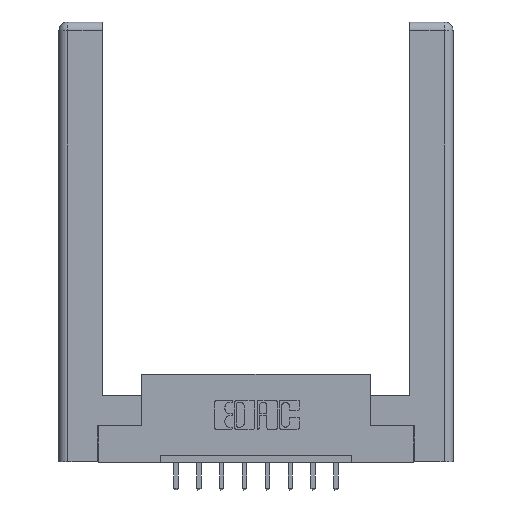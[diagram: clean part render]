
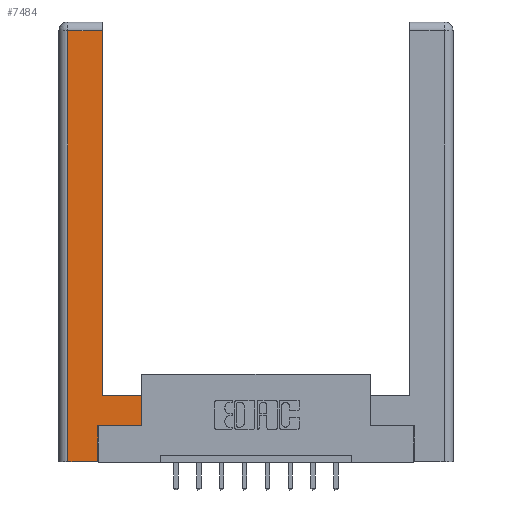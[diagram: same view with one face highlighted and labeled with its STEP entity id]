
A CAD part, top view. The second image highlights one B-rep face of the part: STEP entity #7484.
In plain terms, the highlighted planar face has unit normal (0, 0, 1).
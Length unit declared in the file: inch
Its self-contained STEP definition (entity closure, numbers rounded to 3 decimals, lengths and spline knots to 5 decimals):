
#339 = CARTESIAN_POINT ( 'NONE',  ( 0.295, 3., 0. ) ) ;
#538 = VERTEX_POINT ( 'NONE', #12807 ) ;
#664 = ORIENTED_EDGE ( 'NONE', *, *, #1792, .T. ) ;
#1114 = VERTEX_POINT ( 'NONE', #7267 ) ;
#1497 = EDGE_CURVE ( 'NONE', #6639, #1114, #12967, .T. ) ;
#1628 = EDGE_CURVE ( 'NONE', #7565, #3697, #8568, .T. ) ;
#1708 = VECTOR ( 'NONE', #4663, 39.37008 ) ;
#1780 = CARTESIAN_POINT ( 'NONE',  ( 0.0615, 0., 0. ) ) ;
#1792 = EDGE_CURVE ( 'NONE', #10190, #4879, #8413, .T. ) ;
#1850 = CARTESIAN_POINT ( 'NONE',  ( 0.295, 0.45, 0. ) ) ;
#1873 = VECTOR ( 'NONE', #5642, 39.37008 ) ;
#1914 = DIRECTION ( 'NONE',  ( 0., -1., 0. ) ) ;
#2356 = VECTOR ( 'NONE', #4478, 39.37008 ) ;
#2445 = VECTOR ( 'NONE', #11176, 39.37008 ) ;
#2624 = CARTESIAN_POINT ( 'NONE',  ( 0.565, 0.245, 0. ) ) ;
#2891 = ORIENTED_EDGE ( 'NONE', *, *, #10321, .T. ) ;
#2970 = DIRECTION ( 'NONE',  ( 0., 0., -1. ) ) ;
#3054 = CARTESIAN_POINT ( 'NONE',  ( 0.0615, 2.94, 0. ) ) ;
#3135 = LINE ( 'NONE', #2624, #1708 ) ;
#3470 = CARTESIAN_POINT ( 'NONE',  ( 0.265, 0., 0. ) ) ;
#3697 = VERTEX_POINT ( 'NONE', #6458 ) ;
#3754 = EDGE_CURVE ( 'NONE', #3697, #10190, #5165, .T. ) ;
#3959 = ORIENTED_EDGE ( 'NONE', *, *, #4753, .T. ) ;
#4136 = EDGE_LOOP ( 'NONE', ( #6158, #7349, #664, #9081, #11335, #2891, #3959, #4630 ) ) ;
#4271 = CARTESIAN_POINT ( 'NONE',  ( 0.0615, 2.94, 0. ) ) ;
#4478 = DIRECTION ( 'NONE',  ( -1., 0., 0. ) ) ;
#4630 = ORIENTED_EDGE ( 'NONE', *, *, #10845, .T. ) ;
#4663 = DIRECTION ( 'NONE',  ( 1., 0., 0. ) ) ;
#4753 = EDGE_CURVE ( 'NONE', #538, #11737, #5563, .T. ) ;
#4879 = VERTEX_POINT ( 'NONE', #10035 ) ;
#5082 = VECTOR ( 'NONE', #11844, 39.37008 ) ;
#5165 = LINE ( 'NONE', #3054, #2445 ) ;
#5563 = LINE ( 'NONE', #10769, #1873 ) ;
#5642 = DIRECTION ( 'NONE',  ( 0., 1., 0. ) ) ;
#5874 = VECTOR ( 'NONE', #9494, 39.37008 ) ;
#6158 = ORIENTED_EDGE ( 'NONE', *, *, #1628, .T. ) ;
#6458 = CARTESIAN_POINT ( 'NONE',  ( 0.295, 2.94, 0. ) ) ;
#6639 = VERTEX_POINT ( 'NONE', #3470 ) ;
#6864 = DIRECTION ( 'NONE',  ( 0., 1., 0. ) ) ;
#7267 = CARTESIAN_POINT ( 'NONE',  ( 0.265, 0.245, 0. ) ) ;
#7349 = ORIENTED_EDGE ( 'NONE', *, *, #3754, .T. ) ;
#7484 = ADVANCED_FACE ( 'NONE', ( #10238 ), #11708, .F. ) ;
#7565 = VERTEX_POINT ( 'NONE', #1850 ) ;
#7732 = CARTESIAN_POINT ( 'NONE',  ( 0.565, 0.45, 0. ) ) ;
#7932 = VECTOR ( 'NONE', #6864, 39.37008 ) ;
#8118 = LINE ( 'NONE', #10938, #5082 ) ;
#8413 = LINE ( 'NONE', #1780, #9215 ) ;
#8568 = LINE ( 'NONE', #339, #5874 ) ;
#8913 = CARTESIAN_POINT ( 'NONE',  ( 0.265, 0.245, 0. ) ) ;
#9081 = ORIENTED_EDGE ( 'NONE', *, *, #10480, .T. ) ;
#9215 = VECTOR ( 'NONE', #1914, 39.37008 ) ;
#9494 = DIRECTION ( 'NONE',  ( 0., 1., 0. ) ) ;
#10008 = DIRECTION ( 'NONE',  ( -1., 0., 0. ) ) ;
#10035 = CARTESIAN_POINT ( 'NONE',  ( 0.0615, 0., 0. ) ) ;
#10190 = VERTEX_POINT ( 'NONE', #4271 ) ;
#10238 = FACE_OUTER_BOUND ( 'NONE', #4136, .T. ) ;
#10321 = EDGE_CURVE ( 'NONE', #1114, #538, #3135, .T. ) ;
#10350 = AXIS2_PLACEMENT_3D ( 'NONE', #11792, #2970, #10008 ) ;
#10480 = EDGE_CURVE ( 'NONE', #4879, #6639, #8118, .T. ) ;
#10769 = CARTESIAN_POINT ( 'NONE',  ( 0.565, 0.45, 0. ) ) ;
#10845 = EDGE_CURVE ( 'NONE', #11737, #7565, #11564, .T. ) ;
#10938 = CARTESIAN_POINT ( 'NONE',  ( 0.265, 0., 0. ) ) ;
#11176 = DIRECTION ( 'NONE',  ( -1., 0., 0. ) ) ;
#11335 = ORIENTED_EDGE ( 'NONE', *, *, #1497, .T. ) ;
#11564 = LINE ( 'NONE', #12527, #2356 ) ;
#11708 = PLANE ( 'NONE',  #10350 ) ;
#11737 = VERTEX_POINT ( 'NONE', #7732 ) ;
#11792 = CARTESIAN_POINT ( 'NONE',  ( 0., 0., 0. ) ) ;
#11844 = DIRECTION ( 'NONE',  ( 1., 0., 0. ) ) ;
#12527 = CARTESIAN_POINT ( 'NONE',  ( 0.295, 0.45, 0. ) ) ;
#12807 = CARTESIAN_POINT ( 'NONE',  ( 0.565, 0.245, 0. ) ) ;
#12967 = LINE ( 'NONE', #8913, #7932 ) ;
